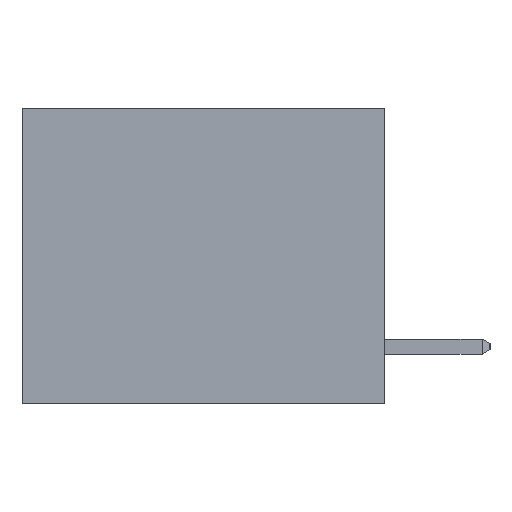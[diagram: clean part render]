
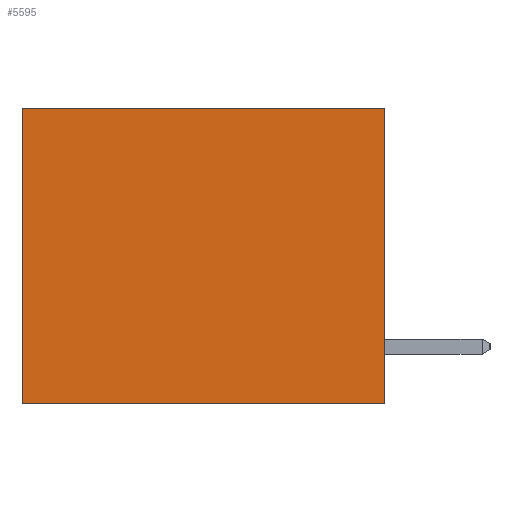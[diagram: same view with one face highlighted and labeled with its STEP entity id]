
A CAD part, left-side view. The second image highlights one B-rep face of the part: STEP entity #5595.
In plain terms, the highlighted planar face has unit normal (-1, 0, 0).
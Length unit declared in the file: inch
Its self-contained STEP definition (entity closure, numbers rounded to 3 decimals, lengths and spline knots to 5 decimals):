
#119 = AXIS2_PLACEMENT_3D ( 'NONE', #2627, #2488, #3713 ) ;
#257 = VECTOR ( 'NONE', #2666, 39.37008 ) ;
#358 = FACE_OUTER_BOUND ( 'NONE', #5574, .T. ) ;
#390 = PLANE ( 'NONE',  #119 ) ;
#403 = CARTESIAN_POINT ( 'NONE',  ( 0.3165, 0.6, 0. ) ) ;
#612 = ORIENTED_EDGE ( 'NONE', *, *, #7949, .F. ) ;
#1588 = CARTESIAN_POINT ( 'NONE',  ( 0.3165, 0., 0. ) ) ;
#1685 = CARTESIAN_POINT ( 'NONE',  ( 0.3165, 0., -0.49 ) ) ;
#2095 = CARTESIAN_POINT ( 'NONE',  ( 0.3165, 0.6, -0.49 ) ) ;
#2269 = CARTESIAN_POINT ( 'NONE',  ( 0.3165, 0., 0. ) ) ;
#2438 = VERTEX_POINT ( 'NONE', #2269 ) ;
#2488 = DIRECTION ( 'NONE',  ( 1., 0., 0. ) ) ;
#2627 = CARTESIAN_POINT ( 'NONE',  ( 0.3165, 0., -0.49 ) ) ;
#2666 = DIRECTION ( 'NONE',  ( 0., 1., 0. ) ) ;
#3272 = CARTESIAN_POINT ( 'NONE',  ( 0.3165, 0., -0.49 ) ) ;
#3322 = VECTOR ( 'NONE', #11612, 39.37008 ) ;
#3713 = DIRECTION ( 'NONE',  ( 0., 0., -1. ) ) ;
#4793 = VECTOR ( 'NONE', #11328, 39.37008 ) ;
#5094 = LINE ( 'NONE', #1588, #257 ) ;
#5574 = EDGE_LOOP ( 'NONE', ( #11219, #612, #6606, #13711 ) ) ;
#5595 = ADVANCED_FACE ( 'NONE', ( #358 ), #390, .F. ) ;
#5641 = VERTEX_POINT ( 'NONE', #6929 ) ;
#6163 = LINE ( 'NONE', #8303, #3322 ) ;
#6606 = ORIENTED_EDGE ( 'NONE', *, *, #8288, .F. ) ;
#6923 = EDGE_CURVE ( 'NONE', #7002, #10223, #6163, .T. ) ;
#6929 = CARTESIAN_POINT ( 'NONE',  ( 0.3165, 0., -0.49 ) ) ;
#7002 = VERTEX_POINT ( 'NONE', #403 ) ;
#7164 = LINE ( 'NONE', #3272, #12698 ) ;
#7949 = EDGE_CURVE ( 'NONE', #5641, #10223, #7164, .T. ) ;
#8288 = EDGE_CURVE ( 'NONE', #2438, #5641, #13542, .T. ) ;
#8303 = CARTESIAN_POINT ( 'NONE',  ( 0.3165, 0.6, -0.49 ) ) ;
#8413 = DIRECTION ( 'NONE',  ( 0., 1., 0. ) ) ;
#10223 = VERTEX_POINT ( 'NONE', #2095 ) ;
#11219 = ORIENTED_EDGE ( 'NONE', *, *, #6923, .T. ) ;
#11328 = DIRECTION ( 'NONE',  ( 0., 0., -1. ) ) ;
#11612 = DIRECTION ( 'NONE',  ( 0., 0., -1. ) ) ;
#12698 = VECTOR ( 'NONE', #8413, 39.37008 ) ;
#12853 = EDGE_CURVE ( 'NONE', #2438, #7002, #5094, .T. ) ;
#13542 = LINE ( 'NONE', #1685, #4793 ) ;
#13711 = ORIENTED_EDGE ( 'NONE', *, *, #12853, .T. ) ;
